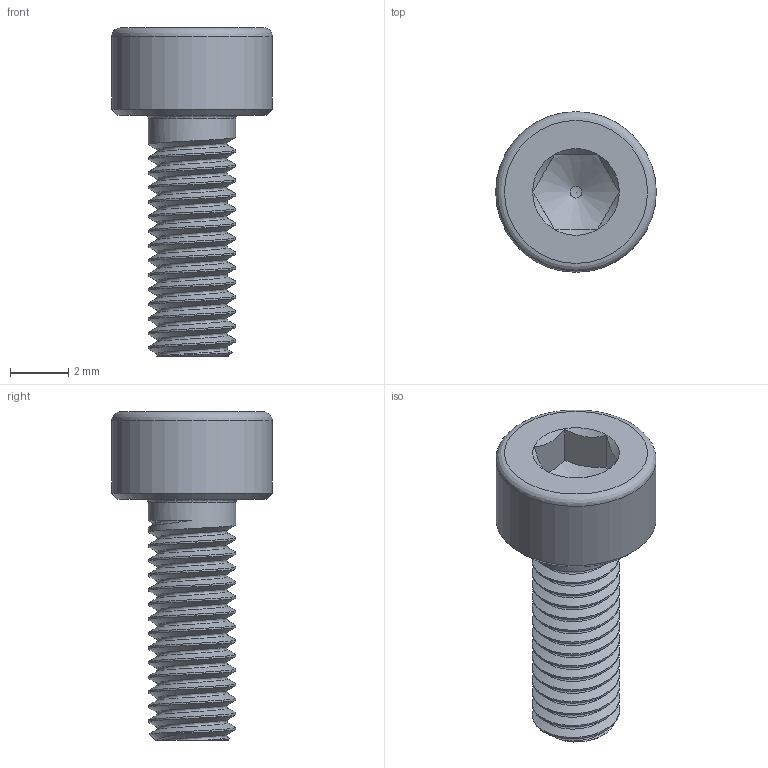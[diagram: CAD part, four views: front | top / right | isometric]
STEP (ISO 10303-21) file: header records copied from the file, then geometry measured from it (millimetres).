
FILE_DESCRIPTION(('FreeCAD Model'),'2;1');
FILE_NAME('Open CASCADE Shape Model','2022-12-07T11:22:12',('Author'),( ''),'Open CASCADE STEP processor 7.6','FreeCAD','Unknown');
FILE_SCHEMA(('AUTOMOTIVE_DESIGN { 1 0 10303 214 1 1 1 1 }'));
Length unit declared in the file: millimetre
Products named in the file (1): M3x8-Screw001
Bounding box: 5.5 x 5.5 x 11.25 mm (x, y, z)
Volume: 109 mm3; surface area: 217.7 mm2
Topology: 1 solids, 1 shells, 81 faces, 200 edges, 121 vertices
Faces by surface type: bspline 48, cylinder 16, plane 9, cone 5, revolution 2, sphere 1
Full cylindrical faces by diameter (mm): 3 x14, 5.5 x1
Entity records: 15181 total; most frequent: CARTESIAN_POINT 12028, ORIENTED_EDGE 396, PCURVE 396, DEFINITIONAL_REPRESENTATION 396, B_SPLINE_CURVE_WITH_KNOTS 339, DIRECTION 309, EDGE_CURVE 198, SURFACE_CURVE 190
